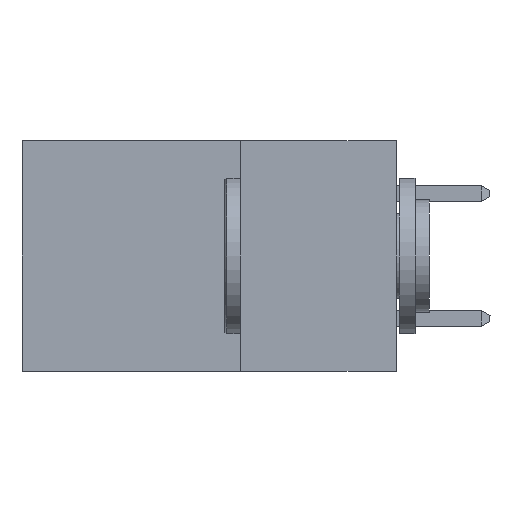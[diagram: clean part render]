
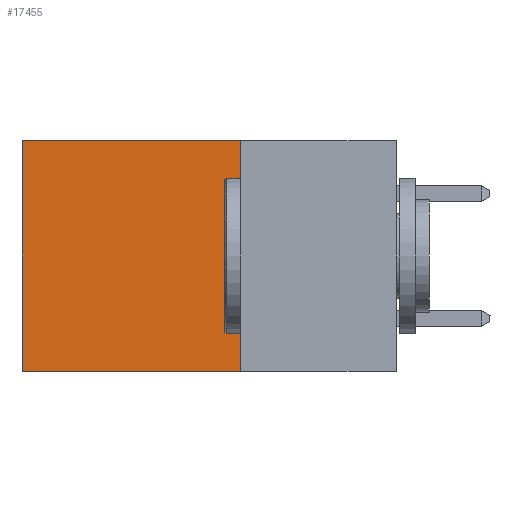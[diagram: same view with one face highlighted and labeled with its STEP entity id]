
A CAD part, left-side view. The second image highlights one B-rep face of the part: STEP entity #17455.
In plain terms, the highlighted planar face has unit normal (-1, 0, 0).
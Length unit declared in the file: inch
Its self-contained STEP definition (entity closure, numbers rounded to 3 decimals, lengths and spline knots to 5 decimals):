
#716 = VECTOR ( 'NONE', #12998, 39.37008 ) ;
#812 = EDGE_CURVE ( 'NONE', #1040, #16955, #17322, .T. ) ;
#1040 = VERTEX_POINT ( 'NONE', #18562 ) ;
#1043 = ORIENTED_EDGE ( 'NONE', *, *, #8364, .T. ) ;
#1100 = CARTESIAN_POINT ( 'NONE',  ( 0.298, 0.6, 0. ) ) ;
#1210 = PLANE ( 'NONE',  #11998 ) ;
#1484 = ORIENTED_EDGE ( 'NONE', *, *, #812, .F. ) ;
#3478 = LINE ( 'NONE', #7941, #6573 ) ;
#4589 = LINE ( 'NONE', #19453, #6018 ) ;
#5701 = DIRECTION ( 'NONE',  ( 1., 0., 0. ) ) ;
#5776 = CARTESIAN_POINT ( 'NONE',  ( 0.298, 0.25, 0. ) ) ;
#6018 = VECTOR ( 'NONE', #10309, 39.37008 ) ;
#6573 = VECTOR ( 'NONE', #8006, 39.37008 ) ;
#7574 = VERTEX_POINT ( 'NONE', #1100 ) ;
#7623 = ORIENTED_EDGE ( 'NONE', *, *, #13966, .F. ) ;
#7941 = CARTESIAN_POINT ( 'NONE',  ( 0.298, 0.6, 0. ) ) ;
#8006 = DIRECTION ( 'NONE',  ( 0., 0., -1. ) ) ;
#8146 = ORIENTED_EDGE ( 'NONE', *, *, #17392, .T. ) ;
#8364 = EDGE_CURVE ( 'NONE', #7574, #16955, #3478, .T. ) ;
#8588 = DIRECTION ( 'NONE',  ( 0., 0., -1. ) ) ;
#9381 = VECTOR ( 'NONE', #13354, 39.37008 ) ;
#10309 = DIRECTION ( 'NONE',  ( 0., 0., -1. ) ) ;
#11125 = CARTESIAN_POINT ( 'NONE',  ( 0.298, 0.25, 0. ) ) ;
#11635 = CARTESIAN_POINT ( 'NONE',  ( 0.298, 0.25, -0.37 ) ) ;
#11998 = AXIS2_PLACEMENT_3D ( 'NONE', #5776, #5701, #8588 ) ;
#12657 = CARTESIAN_POINT ( 'NONE',  ( 0.298, 0.6, -0.37 ) ) ;
#12998 = DIRECTION ( 'NONE',  ( 0., 1., 0. ) ) ;
#13026 = CARTESIAN_POINT ( 'NONE',  ( 0.298, 0.25, 0. ) ) ;
#13354 = DIRECTION ( 'NONE',  ( 0., 1., 0. ) ) ;
#13966 = EDGE_CURVE ( 'NONE', #14444, #1040, #4589, .T. ) ;
#14444 = VERTEX_POINT ( 'NONE', #11125 ) ;
#16955 = VERTEX_POINT ( 'NONE', #12657 ) ;
#17322 = LINE ( 'NONE', #11635, #716 ) ;
#17392 = EDGE_CURVE ( 'NONE', #14444, #7574, #19623, .T. ) ;
#17455 = ADVANCED_FACE ( 'NONE', ( #18657 ), #1210, .F. ) ;
#18562 = CARTESIAN_POINT ( 'NONE',  ( 0.298, 0.25, -0.37 ) ) ;
#18657 = FACE_OUTER_BOUND ( 'NONE', #19538, .T. ) ;
#19453 = CARTESIAN_POINT ( 'NONE',  ( 0.298, 0.25, 0. ) ) ;
#19538 = EDGE_LOOP ( 'NONE', ( #1043, #1484, #7623, #8146 ) ) ;
#19623 = LINE ( 'NONE', #13026, #9381 ) ;
